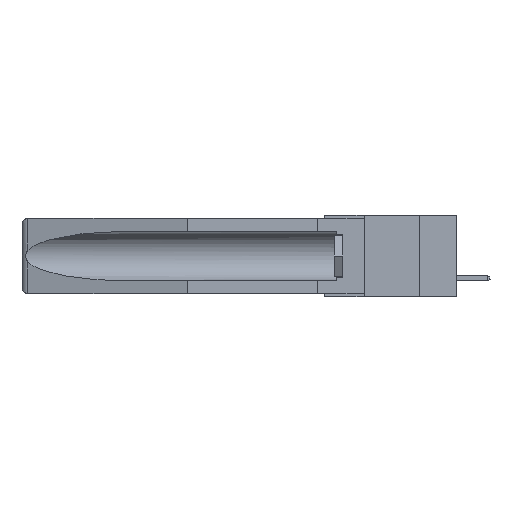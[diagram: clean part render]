
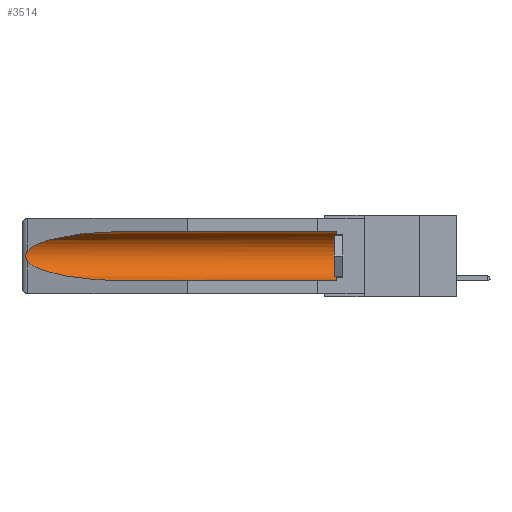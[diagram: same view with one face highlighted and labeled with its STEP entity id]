
A CAD part, left-side view. The second image highlights one B-rep face of the part: STEP entity #3514.
In plain terms, the highlighted cylindrical face has radius 2.857 mm (diameter 5.715 mm), a partial arc.
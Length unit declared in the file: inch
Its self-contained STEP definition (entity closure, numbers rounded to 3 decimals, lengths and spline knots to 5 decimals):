
#211 = DIRECTION ( 'NONE',  ( 0., 1., 0. ) ) ;
#1306 = CARTESIAN_POINT ( 'NONE',  ( 0.2675, 1.53308, -0.16763 ) ) ;
#1333 = CARTESIAN_POINT ( 'NONE',  ( 0.155, 0.126, -0.059 ) ) ;
#1504 = VECTOR ( 'NONE', #8602, 39.37008 ) ;
#2206 = DIRECTION ( 'NONE',  ( 0., 1., 0. ) ) ;
#2577 = ORIENTED_EDGE ( 'NONE', *, *, #9121, .T. ) ;
#2609 = DIRECTION ( 'NONE',  ( 0., 0., 1. ) ) ;
#2963 = EDGE_CURVE ( 'NONE', #11250, #10510, #5854, .T. ) ;
#3152 =( BOUNDED_CURVE ( )  B_SPLINE_CURVE ( 3, ( #8358, #5848, #3298, #9466 ),
 .UNSPECIFIED., .F., .F. ) 
 B_SPLINE_CURVE_WITH_KNOTS ( ( 4, 4 ),
 ( 0.1948, 1.5708 ),
 .UNSPECIFIED. ) 
 CURVE ( )  GEOMETRIC_REPRESENTATION_ITEM ( )  RATIONAL_B_SPLINE_CURVE ( ( 1., 0.848, 0.848, 1. ) ) 
 REPRESENTATION_ITEM ( '' )  );
#3298 = CARTESIAN_POINT ( 'NONE',  ( 0.21114, 1.30732, -0.284 ) ) ;
#3514 = ADVANCED_FACE ( 'NONE', ( #12407 ), #11076, .F. ) ;
#3863 = CARTESIAN_POINT ( 'NONE',  ( 0.26597, 1.5296, -0.19026 ) ) ;
#3918 = CIRCLE ( 'NONE', #11591, 0.1125 ) ;
#4082 = AXIS2_PLACEMENT_3D ( 'NONE', #13314, #2206, #10875 ) ;
#4883 = VERTEX_POINT ( 'NONE', #14350 ) ;
#4893 = CARTESIAN_POINT ( 'NONE',  ( 0.155, -0.30754, -0.284 ) ) ;
#5268 = CARTESIAN_POINT ( 'NONE',  ( 0.155, 0.126, -0.1715 ) ) ;
#5362 = CARTESIAN_POINT ( 'NONE',  ( 0.155, 1.07973, -0.059 ) ) ;
#5481 = CARTESIAN_POINT ( 'NONE',  ( 0.21114, 1.30732, -0.059 ) ) ;
#5848 = CARTESIAN_POINT ( 'NONE',  ( 0.25451, 1.48313, -0.24835 ) ) ;
#5854 = LINE ( 'NONE', #8821, #6629 ) ;
#6038 = B_SPLINE_CURVE_WITH_KNOTS ( 'NONE', 3,
 ( #12405, #7505, #8757, #7558, #1306, #9977, #11236, #13724, #3863, #13875 ),
 .UNSPECIFIED., .F., .F.,
 ( 4, 2, 2, 2, 4 ),
 ( 0., 0.00029, 0.00058, 0.00087, 0.00117 ),
 .UNSPECIFIED. ) ;
#6318 = ORIENTED_EDGE ( 'NONE', *, *, #7214, .T. ) ;
#6559 = CARTESIAN_POINT ( 'NONE',  ( 0.155, 1.07973, -0.284 ) ) ;
#6629 = VECTOR ( 'NONE', #211, 39.37008 ) ;
#6747 = VERTEX_POINT ( 'NONE', #6559 ) ;
#6935 = CARTESIAN_POINT ( 'NONE',  ( 0.26537, 1.52718, -0.19328 ) ) ;
#7214 = EDGE_CURVE ( 'NONE', #10510, #4883, #8923, .T. ) ;
#7505 = CARTESIAN_POINT ( 'NONE',  ( 0.26597, 1.52961, -0.15275 ) ) ;
#7558 = CARTESIAN_POINT ( 'NONE',  ( 0.2673, 1.5327, -0.16383 ) ) ;
#7655 = EDGE_CURVE ( 'NONE', #4883, #10039, #6038, .T. ) ;
#7813 = CARTESIAN_POINT ( 'NONE',  ( 0.25451, 1.48313, -0.09465 ) ) ;
#8358 = CARTESIAN_POINT ( 'NONE',  ( 0.26537, 1.52718, -0.19328 ) ) ;
#8602 = DIRECTION ( 'NONE',  ( 0., 1., 0. ) ) ;
#8757 = CARTESIAN_POINT ( 'NONE',  ( 0.26654, 1.53092, -0.15636 ) ) ;
#8821 = CARTESIAN_POINT ( 'NONE',  ( 0.155, -0.30754, -0.059 ) ) ;
#8923 =( BOUNDED_CURVE ( )  B_SPLINE_CURVE ( 3, ( #9109, #5481, #7813, #14181 ),
 .UNSPECIFIED., .F., .F. ) 
 B_SPLINE_CURVE_WITH_KNOTS ( ( 4, 4 ),
 ( 4.71239, 6.08839 ),
 .UNSPECIFIED. ) 
 CURVE ( )  GEOMETRIC_REPRESENTATION_ITEM ( )  RATIONAL_B_SPLINE_CURVE ( ( 1., 0.848, 0.848, 1. ) ) 
 REPRESENTATION_ITEM ( '' )  );
#9109 = CARTESIAN_POINT ( 'NONE',  ( 0.155, 1.07973, -0.059 ) ) ;
#9121 = EDGE_CURVE ( 'NONE', #12106, #11250, #3918, .T. ) ;
#9318 = EDGE_CURVE ( 'NONE', #10039, #6747, #3152, .T. ) ;
#9466 = CARTESIAN_POINT ( 'NONE',  ( 0.155, 1.07973, -0.284 ) ) ;
#9654 = LINE ( 'NONE', #4893, #1504 ) ;
#9727 = CARTESIAN_POINT ( 'NONE',  ( 0.155, 0.126, -0.284 ) ) ;
#9977 = CARTESIAN_POINT ( 'NONE',  ( 0.2675, 1.53308, -0.17534 ) ) ;
#10039 = VERTEX_POINT ( 'NONE', #6935 ) ;
#10481 = ORIENTED_EDGE ( 'NONE', *, *, #2963, .T. ) ;
#10510 = VERTEX_POINT ( 'NONE', #5362 ) ;
#10875 = DIRECTION ( 'NONE',  ( 0., 0., 1. ) ) ;
#11076 = CYLINDRICAL_SURFACE ( 'NONE', #4082, 0.1125 ) ;
#11123 = ORIENTED_EDGE ( 'NONE', *, *, #12298, .F. ) ;
#11236 = CARTESIAN_POINT ( 'NONE',  ( 0.2673, 1.53269, -0.17917 ) ) ;
#11250 = VERTEX_POINT ( 'NONE', #1333 ) ;
#11591 = AXIS2_PLACEMENT_3D ( 'NONE', #5268, #12462, #2609 ) ;
#12106 = VERTEX_POINT ( 'NONE', #9727 ) ;
#12298 = EDGE_CURVE ( 'NONE', #12106, #6747, #9654, .T. ) ;
#12405 = CARTESIAN_POINT ( 'NONE',  ( 0.26537, 1.52718, -0.14972 ) ) ;
#12407 = FACE_OUTER_BOUND ( 'NONE', #12530, .T. ) ;
#12462 = DIRECTION ( 'NONE',  ( 0., -1., 0. ) ) ;
#12530 = EDGE_LOOP ( 'NONE', ( #6318, #13131, #15425, #11123, #2577, #10481 ) ) ;
#13131 = ORIENTED_EDGE ( 'NONE', *, *, #7655, .T. ) ;
#13314 = CARTESIAN_POINT ( 'NONE',  ( 0.155, -0.30754, -0.1715 ) ) ;
#13724 = CARTESIAN_POINT ( 'NONE',  ( 0.26655, 1.53094, -0.18657 ) ) ;
#13875 = CARTESIAN_POINT ( 'NONE',  ( 0.26537, 1.52718, -0.19328 ) ) ;
#14181 = CARTESIAN_POINT ( 'NONE',  ( 0.26537, 1.52718, -0.14972 ) ) ;
#14350 = CARTESIAN_POINT ( 'NONE',  ( 0.26537, 1.52718, -0.14972 ) ) ;
#15425 = ORIENTED_EDGE ( 'NONE', *, *, #9318, .T. ) ;
